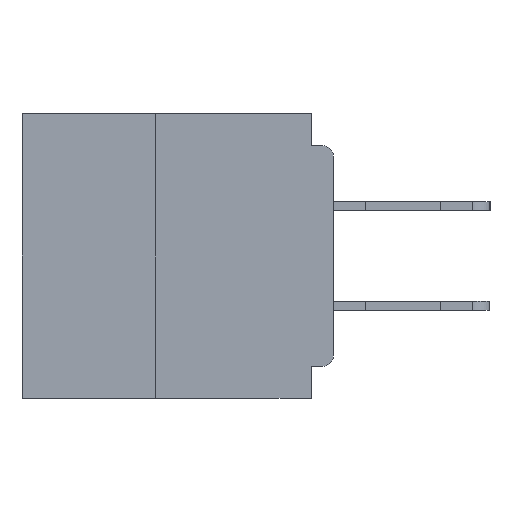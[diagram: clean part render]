
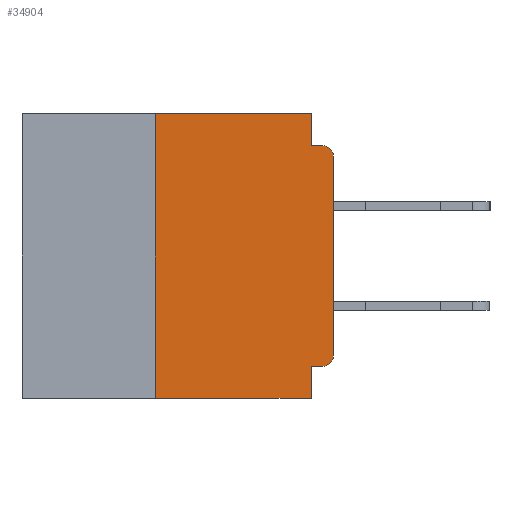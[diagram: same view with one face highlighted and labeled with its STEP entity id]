
A CAD part, left-side view. The second image highlights one B-rep face of the part: STEP entity #34904.
In plain terms, the highlighted planar face has unit normal (-1, 0, 0).
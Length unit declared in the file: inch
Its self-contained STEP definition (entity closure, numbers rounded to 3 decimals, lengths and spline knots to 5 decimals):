
#2227 = LINE ( 'NONE', #39638, #29605 ) ;
#2534 = DIRECTION ( 'NONE',  ( 0., 0., -1. ) ) ;
#3176 = LINE ( 'NONE', #14844, #36180 ) ;
#4166 = VECTOR ( 'NONE', #7257, 39.37008 ) ;
#4727 = CARTESIAN_POINT ( 'NONE',  ( 0., 0.031, -0.045 ) ) ;
#4781 = CARTESIAN_POINT ( 'NONE',  ( 0., 0., -0.355 ) ) ;
#5232 = DIRECTION ( 'NONE',  ( -1., 0., 0. ) ) ;
#5725 = LINE ( 'NONE', #31820, #22249 ) ;
#6433 = EDGE_CURVE ( 'NONE', #39273, #38543, #35346, .T. ) ;
#7257 = DIRECTION ( 'NONE',  ( 0., -1., 0. ) ) ;
#8139 = DIRECTION ( 'NONE',  ( 0., 1., 0. ) ) ;
#9039 = CARTESIAN_POINT ( 'NONE',  ( 0., 0.437, 0. ) ) ;
#9073 = VECTOR ( 'NONE', #37174, 39.37008 ) ;
#9342 = CARTESIAN_POINT ( 'NONE',  ( 0., 0.25, 0. ) ) ;
#10055 = EDGE_CURVE ( 'NONE', #23594, #41426, #33833, .T. ) ;
#10154 = ORIENTED_EDGE ( 'NONE', *, *, #28457, .T. ) ;
#10999 = EDGE_CURVE ( 'NONE', #24073, #16183, #21885, .T. ) ;
#11472 = CARTESIAN_POINT ( 'NONE',  ( 0., 0.015, -0.045 ) ) ;
#12076 = DIRECTION ( 'NONE',  ( 0., -1., 0. ) ) ;
#12726 = ORIENTED_EDGE ( 'NONE', *, *, #6433, .F. ) ;
#12912 = CIRCLE ( 'NONE', #41655, 0.015 ) ;
#12974 = LINE ( 'NONE', #30293, #4166 ) ;
#13424 = EDGE_CURVE ( 'NONE', #35427, #37088, #12912, .T. ) ;
#13517 = CARTESIAN_POINT ( 'NONE',  ( 0., 0.031, 0. ) ) ;
#14543 = ORIENTED_EDGE ( 'NONE', *, *, #10055, .F. ) ;
#14844 = CARTESIAN_POINT ( 'NONE',  ( 0., 0., -0.045 ) ) ;
#15060 = CARTESIAN_POINT ( 'NONE',  ( 0., 0.015, -0.355 ) ) ;
#15548 = DIRECTION ( 'NONE',  ( -1., 0., 0. ) ) ;
#16183 = VERTEX_POINT ( 'NONE', #11472 ) ;
#16631 = CARTESIAN_POINT ( 'NONE',  ( 0., 0.25, -0.4 ) ) ;
#16811 = VERTEX_POINT ( 'NONE', #4727 ) ;
#17261 = FACE_OUTER_BOUND ( 'NONE', #35907, .T. ) ;
#18449 = CARTESIAN_POINT ( 'NONE',  ( 0., 0.031, 0. ) ) ;
#18802 = EDGE_CURVE ( 'NONE', #16811, #16183, #3176, .T. ) ;
#18920 = EDGE_CURVE ( 'NONE', #41426, #41623, #5725, .T. ) ;
#19399 = ORIENTED_EDGE ( 'NONE', *, *, #32686, .F. ) ;
#19946 = DIRECTION ( 'NONE',  ( 0., 0., 1. ) ) ;
#21257 = CARTESIAN_POINT ( 'NONE',  ( 0., 0., -0.06 ) ) ;
#21710 = DIRECTION ( 'NONE',  ( 0., 0., -1. ) ) ;
#21882 = EDGE_CURVE ( 'NONE', #23594, #38543, #12974, .T. ) ;
#21885 = CIRCLE ( 'NONE', #30619, 0.015 ) ;
#22157 = ORIENTED_EDGE ( 'NONE', *, *, #18920, .F. ) ;
#22249 = VECTOR ( 'NONE', #12076, 39.37008 ) ;
#22281 = DIRECTION ( 'NONE',  ( 1., 0., 0. ) ) ;
#23594 = VERTEX_POINT ( 'NONE', #41812 ) ;
#23939 = CARTESIAN_POINT ( 'NONE',  ( 0., 0.031, -0.4 ) ) ;
#24039 = VECTOR ( 'NONE', #39626, 39.37008 ) ;
#24073 = VERTEX_POINT ( 'NONE', #21257 ) ;
#24608 = ORIENTED_EDGE ( 'NONE', *, *, #35360, .F. ) ;
#24996 = CARTESIAN_POINT ( 'NONE',  ( 0., 0.015, -0.34 ) ) ;
#28076 = CARTESIAN_POINT ( 'NONE',  ( 0., 0.031, -0.355 ) ) ;
#28299 = DIRECTION ( 'NONE',  ( 0., 0., -1. ) ) ;
#28457 = EDGE_CURVE ( 'NONE', #37088, #24073, #2227, .T. ) ;
#29605 = VECTOR ( 'NONE', #19946, 39.37008 ) ;
#29978 = ORIENTED_EDGE ( 'NONE', *, *, #10999, .T. ) ;
#30293 = CARTESIAN_POINT ( 'NONE',  ( 0., 0.437, -0.4 ) ) ;
#30619 = AXIS2_PLACEMENT_3D ( 'NONE', #35252, #15548, #38550 ) ;
#30646 = ORIENTED_EDGE ( 'NONE', *, *, #21882, .T. ) ;
#31070 = ORIENTED_EDGE ( 'NONE', *, *, #18802, .F. ) ;
#31820 = CARTESIAN_POINT ( 'NONE',  ( 0., 0.437, 0. ) ) ;
#32686 = EDGE_CURVE ( 'NONE', #41623, #16811, #33917, .T. ) ;
#33833 = LINE ( 'NONE', #16631, #24039 ) ;
#33917 = LINE ( 'NONE', #18449, #42608 ) ;
#34904 = ADVANCED_FACE ( 'NONE', ( #17261 ), #41941, .F. ) ;
#35252 = CARTESIAN_POINT ( 'NONE',  ( 0., 0.015, -0.06 ) ) ;
#35346 = LINE ( 'NONE', #23939, #9073 ) ;
#35360 = EDGE_CURVE ( 'NONE', #35427, #39273, #41340, .T. ) ;
#35427 = VERTEX_POINT ( 'NONE', #15060 ) ;
#35672 = ORIENTED_EDGE ( 'NONE', *, *, #13424, .T. ) ;
#35907 = EDGE_LOOP ( 'NONE', ( #10154, #29978, #31070, #19399, #22157, #14543, #30646, #12726, #24608, #35672 ) ) ;
#36180 = VECTOR ( 'NONE', #37842, 39.37008 ) ;
#36189 = CARTESIAN_POINT ( 'NONE',  ( 0., 0., -0.34 ) ) ;
#37088 = VERTEX_POINT ( 'NONE', #36189 ) ;
#37174 = DIRECTION ( 'NONE',  ( 0., 0., -1. ) ) ;
#37842 = DIRECTION ( 'NONE',  ( 0., -1., 0. ) ) ;
#38543 = VERTEX_POINT ( 'NONE', #40354 ) ;
#38550 = DIRECTION ( 'NONE',  ( 0., 0., -1. ) ) ;
#39273 = VERTEX_POINT ( 'NONE', #28076 ) ;
#39626 = DIRECTION ( 'NONE',  ( 0., 0., 1. ) ) ;
#39638 = CARTESIAN_POINT ( 'NONE',  ( 0., 0., 0. ) ) ;
#39781 = AXIS2_PLACEMENT_3D ( 'NONE', #9039, #22281, #2534 ) ;
#40339 = VECTOR ( 'NONE', #8139, 39.37008 ) ;
#40354 = CARTESIAN_POINT ( 'NONE',  ( 0., 0.031, -0.4 ) ) ;
#41340 = LINE ( 'NONE', #4781, #40339 ) ;
#41426 = VERTEX_POINT ( 'NONE', #9342 ) ;
#41623 = VERTEX_POINT ( 'NONE', #13517 ) ;
#41655 = AXIS2_PLACEMENT_3D ( 'NONE', #24996, #5232, #28299 ) ;
#41812 = CARTESIAN_POINT ( 'NONE',  ( 0., 0.25, -0.4 ) ) ;
#41941 = PLANE ( 'NONE',  #39781 ) ;
#42608 = VECTOR ( 'NONE', #21710, 39.37008 ) ;
